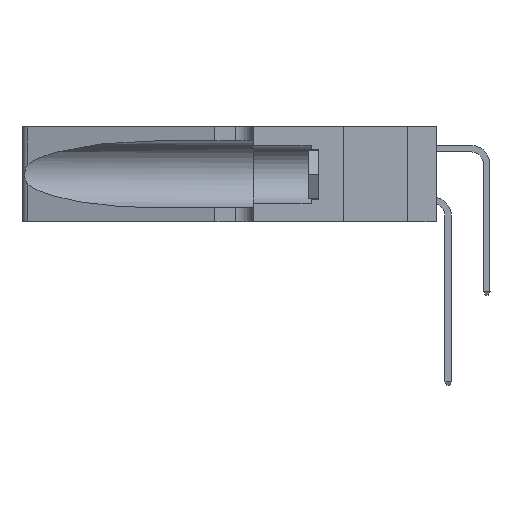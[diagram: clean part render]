
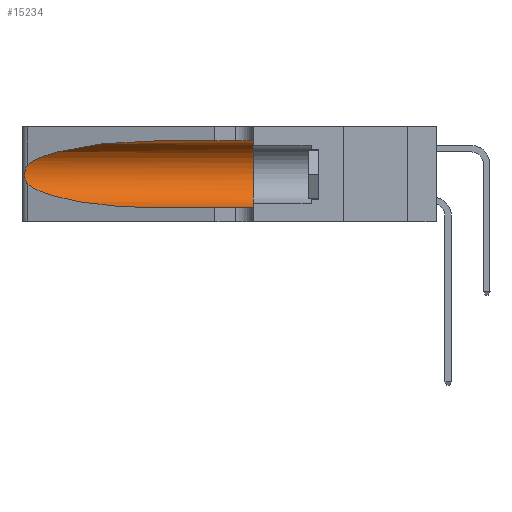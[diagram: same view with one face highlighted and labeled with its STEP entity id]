
A CAD part, left-side view. The second image highlights one B-rep face of the part: STEP entity #15234.
In plain terms, the highlighted cylindrical face has radius 3.308 mm (diameter 6.617 mm), a partial arc.
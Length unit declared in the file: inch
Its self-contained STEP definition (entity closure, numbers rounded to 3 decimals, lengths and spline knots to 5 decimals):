
#946 = CARTESIAN_POINT ( 'NONE',  ( 0.1305, 0.72297, 0.05475 ) ) ;
#1549 = ORIENTED_EDGE ( 'NONE', *, *, #43165, .F. ) ;
#1580 = CARTESIAN_POINT ( 'NONE',  ( 0.25639, 1.23184, 0.21858 ) ) ;
#1731 = DIRECTION ( 'NONE',  ( 0., 1., 0. ) ) ;
#2432 = DIRECTION ( 'NONE',  ( 0., 0., -1. ) ) ;
#3581 = EDGE_CURVE ( 'NONE', #9377, #32932, #8416, .T. ) ;
#4073 = EDGE_CURVE ( 'NONE', #41318, #9377, #36676, .T. ) ;
#5051 = CARTESIAN_POINT ( 'NONE',  ( 0.25854, 1.2359, 0.20912 ) ) ;
#5079 = CARTESIAN_POINT ( 'NONE',  ( 0.1305, 0.35, 0.05475 ) ) ;
#5093 =( BOUNDED_CURVE ( )  B_SPLINE_CURVE ( 3, ( #17979, #28111, #21375, #946 ),
 .UNSPECIFIED., .F., .F. ) 
 B_SPLINE_CURVE_WITH_KNOTS ( ( 4, 4 ),
 ( 3.44316, 4.71239 ),
 .UNSPECIFIED. ) 
 CURVE ( )  GEOMETRIC_REPRESENTATION_ITEM ( )  RATIONAL_B_SPLINE_CURVE ( ( 1., 0.87, 0.87, 1. ) ) 
 REPRESENTATION_ITEM ( '' )  );
#5940 = ORIENTED_EDGE ( 'NONE', *, *, #7249, .T. ) ;
#5961 = CARTESIAN_POINT ( 'NONE',  ( 0.1305, 0.72297, 0.31525 ) ) ;
#7249 = EDGE_CURVE ( 'NONE', #32932, #32991, #5093, .T. ) ;
#7576 = EDGE_LOOP ( 'NONE', ( #27377, #22370, #5940, #24592, #1549, #27778 ) ) ;
#7877 = CARTESIAN_POINT ( 'NONE',  ( 0.1305, 0.72297, 0.31525 ) ) ;
#8416 = B_SPLINE_CURVE_WITH_KNOTS ( 'NONE', 3,
 ( #21992, #42320, #1580, #25435, #5051, #28860, #8515, #32255, #11914, #35634, #15332, #39093, #18729, #42461 ),
 .UNSPECIFIED., .F., .F.,
 ( 4, 2, 2, 2, 2, 2, 4 ),
 ( 0., 0.00027, 0.00053, 0.00107, 0.0016, 0.00187, 0.00214 ),
 .UNSPECIFIED. ) ;
#8515 = CARTESIAN_POINT ( 'NONE',  ( 0.26075, 1.23896, 0.19203 ) ) ;
#9377 = VERTEX_POINT ( 'NONE', #25945 ) ;
#11887 = CYLINDRICAL_SURFACE ( 'NONE', #32623, 0.13025 ) ;
#11914 = CARTESIAN_POINT ( 'NONE',  ( 0.26017, 1.23833, 0.17102 ) ) ;
#13335 = LINE ( 'NONE', #27045, #39376 ) ;
#14412 = VERTEX_POINT ( 'NONE', #5079 ) ;
#15159 = EDGE_CURVE ( 'NONE', #32991, #14412, #34659, .T. ) ;
#15234 = ADVANCED_FACE ( 'NONE', ( #29962 ), #11887, .F. ) ;
#15332 = CARTESIAN_POINT ( 'NONE',  ( 0.25789, 1.23486, 0.15765 ) ) ;
#16465 = CARTESIAN_POINT ( 'NONE',  ( 0.1305, 0.72297, 0.05475 ) ) ;
#16765 = EDGE_CURVE ( 'NONE', #41318, #18589, #13335, .T. ) ;
#17979 = CARTESIAN_POINT ( 'NONE',  ( 0.25487, 1.22718, 0.14631 ) ) ;
#18096 = CARTESIAN_POINT ( 'NONE',  ( 0.25487, 1.22718, 0.22369 ) ) ;
#18589 = VERTEX_POINT ( 'NONE', #26614 ) ;
#18729 = CARTESIAN_POINT ( 'NONE',  ( 0.25555, 1.22993, 0.14849 ) ) ;
#21375 = CARTESIAN_POINT ( 'NONE',  ( 0.18966, 0.96281, 0.05475 ) ) ;
#21992 = CARTESIAN_POINT ( 'NONE',  ( 0.25487, 1.22718, 0.22369 ) ) ;
#22150 = CARTESIAN_POINT ( 'NONE',  ( 0.1305, 0.35, 0.185 ) ) ;
#22370 = ORIENTED_EDGE ( 'NONE', *, *, #3581, .T. ) ;
#22855 = CARTESIAN_POINT ( 'NONE',  ( 0.1305, 1.61858, 0.185 ) ) ;
#24592 = ORIENTED_EDGE ( 'NONE', *, *, #15159, .T. ) ;
#24797 = CARTESIAN_POINT ( 'NONE',  ( 0.18966, 0.96281, 0.31525 ) ) ;
#25435 = CARTESIAN_POINT ( 'NONE',  ( 0.25787, 1.23484, 0.2124 ) ) ;
#25581 = DIRECTION ( 'NONE',  ( 0., 0., 1. ) ) ;
#25945 = CARTESIAN_POINT ( 'NONE',  ( 0.25487, 1.22718, 0.22369 ) ) ;
#26614 = CARTESIAN_POINT ( 'NONE',  ( 0.1305, 0.35, 0.31525 ) ) ;
#27045 = CARTESIAN_POINT ( 'NONE',  ( 0.1305, 1.61858, 0.31525 ) ) ;
#27377 = ORIENTED_EDGE ( 'NONE', *, *, #4073, .T. ) ;
#27778 = ORIENTED_EDGE ( 'NONE', *, *, #16765, .F. ) ;
#28111 = CARTESIAN_POINT ( 'NONE',  ( 0.2373, 1.15595, 0.08982 ) ) ;
#28477 = AXIS2_PLACEMENT_3D ( 'NONE', #22150, #1731, #25581 ) ;
#28860 = CARTESIAN_POINT ( 'NONE',  ( 0.26018, 1.23835, 0.19895 ) ) ;
#29962 = FACE_OUTER_BOUND ( 'NONE', #7576, .T. ) ;
#32255 = CARTESIAN_POINT ( 'NONE',  ( 0.26075, 1.23896, 0.178 ) ) ;
#32623 = AXIS2_PLACEMENT_3D ( 'NONE', #22855, #36343, #2432 ) ;
#32932 = VERTEX_POINT ( 'NONE', #43304 ) ;
#32991 = VERTEX_POINT ( 'NONE', #16465 ) ;
#33588 = VECTOR ( 'NONE', #42720, 39.37008 ) ;
#34659 = LINE ( 'NONE', #35903, #33588 ) ;
#35634 = CARTESIAN_POINT ( 'NONE',  ( 0.25856, 1.23593, 0.16098 ) ) ;
#35903 = CARTESIAN_POINT ( 'NONE',  ( 0.1305, 1.61858, 0.05475 ) ) ;
#36343 = DIRECTION ( 'NONE',  ( 0., -1., 0. ) ) ;
#36676 =( BOUNDED_CURVE ( )  B_SPLINE_CURVE ( 3, ( #7877, #24797, #38446, #18096 ),
 .UNSPECIFIED., .F., .T. ) 
 B_SPLINE_CURVE_WITH_KNOTS ( ( 4, 4 ),
 ( 1.5708, 2.84003 ),
 .UNSPECIFIED. ) 
 CURVE ( )  GEOMETRIC_REPRESENTATION_ITEM ( )  RATIONAL_B_SPLINE_CURVE ( ( 1., 0.87, 0.87, 1. ) ) 
 REPRESENTATION_ITEM ( '' )  );
#37274 = DIRECTION ( 'NONE',  ( 0., -1., 0. ) ) ;
#38446 = CARTESIAN_POINT ( 'NONE',  ( 0.2373, 1.15595, 0.28018 ) ) ;
#39093 = CARTESIAN_POINT ( 'NONE',  ( 0.25639, 1.23186, 0.15144 ) ) ;
#39376 = VECTOR ( 'NONE', #37274, 39.37008 ) ;
#40421 = CIRCLE ( 'NONE', #28477, 0.13025 ) ;
#41318 = VERTEX_POINT ( 'NONE', #5961 ) ;
#42320 = CARTESIAN_POINT ( 'NONE',  ( 0.25555, 1.22994, 0.2215 ) ) ;
#42461 = CARTESIAN_POINT ( 'NONE',  ( 0.25487, 1.22718, 0.14631 ) ) ;
#42720 = DIRECTION ( 'NONE',  ( 0., -1., 0. ) ) ;
#43165 = EDGE_CURVE ( 'NONE', #18589, #14412, #40421, .T. ) ;
#43304 = CARTESIAN_POINT ( 'NONE',  ( 0.25487, 1.22718, 0.14631 ) ) ;
